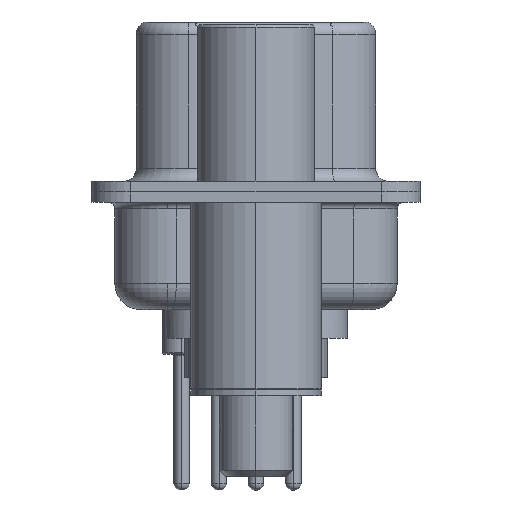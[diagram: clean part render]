
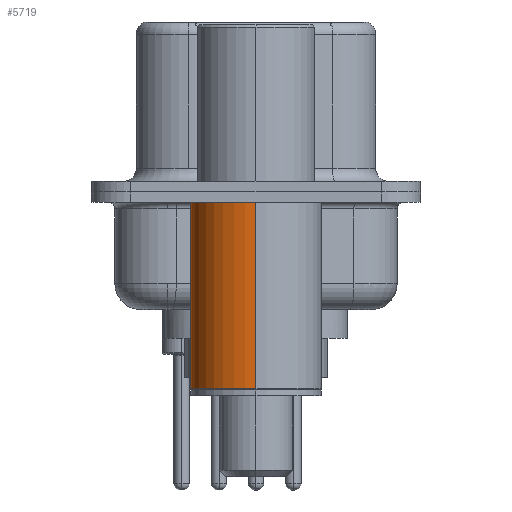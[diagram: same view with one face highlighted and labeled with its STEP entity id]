
A CAD part, left-side view. The second image highlights one B-rep face of the part: STEP entity #5719.
In plain terms, the highlighted cylindrical face has radius 2.5 mm (diameter 5 mm), a partial arc.
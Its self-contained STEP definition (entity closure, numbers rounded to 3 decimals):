
#463 = ORIENTED_EDGE ( 'NONE', *, *, #3000, .F. ) ;
#952 = DIRECTION ( 'NONE',  ( 0., 0., 1. ) ) ;
#1108 = CARTESIAN_POINT ( 'NONE',  ( 2.5, 0., 0.581 ) ) ;
#1246 = FACE_OUTER_BOUND ( 'NONE', #25234, .T. ) ;
#1771 = CIRCLE ( 'NONE', #19673, 2.5 ) ;
#1999 = VECTOR ( 'NONE', #24721, 1000. ) ;
#2652 = LINE ( 'NONE', #24866, #1999 ) ;
#2879 = DIRECTION ( 'NONE',  ( 1., 0., 0. ) ) ;
#3000 = EDGE_CURVE ( 'NONE', #19022, #24059, #10013, .T. ) ;
#3647 = DIRECTION ( 'NONE',  ( 1., 0., 0. ) ) ;
#4002 = EDGE_CURVE ( 'NONE', #20399, #24059, #2652, .T. ) ;
#4532 = EDGE_CURVE ( 'NONE', #15777, #19022, #20188, .T. ) ;
#5174 = CARTESIAN_POINT ( 'NONE',  ( 0., 0., -0.4 ) ) ;
#5719 = ADVANCED_FACE ( 'NONE', ( #1246 ), #17496, .T. ) ;
#7270 = CARTESIAN_POINT ( 'NONE',  ( 0., 0., -7.525 ) ) ;
#7713 = ORIENTED_EDGE ( 'NONE', *, *, #18188, .T. ) ;
#9398 = DIRECTION ( 'NONE',  ( 1., 0., 0. ) ) ;
#9495 = DIRECTION ( 'NONE',  ( 0., 0., 1. ) ) ;
#9958 = CARTESIAN_POINT ( 'NONE',  ( -2.5, 0., -7.525 ) ) ;
#10013 = CIRCLE ( 'NONE', #23961, 2.5 ) ;
#11691 = ORIENTED_EDGE ( 'NONE', *, *, #4532, .F. ) ;
#12220 = DIRECTION ( 'NONE',  ( 0., 0., 1. ) ) ;
#12671 = CARTESIAN_POINT ( 'NONE',  ( 2.5, 0., -0.4 ) ) ;
#15777 = VERTEX_POINT ( 'NONE', #18247 ) ;
#16660 = ORIENTED_EDGE ( 'NONE', *, *, #4002, .T. ) ;
#17496 = CYLINDRICAL_SURFACE ( 'NONE', #27222, 2.5 ) ;
#18188 = EDGE_CURVE ( 'NONE', #15777, #20399, #1771, .T. ) ;
#18247 = CARTESIAN_POINT ( 'NONE',  ( 2.5, 0., -7.525 ) ) ;
#18880 = VECTOR ( 'NONE', #952, 1000. ) ;
#19022 = VERTEX_POINT ( 'NONE', #12671 ) ;
#19673 = AXIS2_PLACEMENT_3D ( 'NONE', #7270, #22057, #9398 ) ;
#20188 = LINE ( 'NONE', #1108, #18880 ) ;
#20399 = VERTEX_POINT ( 'NONE', #9958 ) ;
#22057 = DIRECTION ( 'NONE',  ( 0., 0., 1. ) ) ;
#23961 = AXIS2_PLACEMENT_3D ( 'NONE', #5174, #9495, #2879 ) ;
#24059 = VERTEX_POINT ( 'NONE', #24140 ) ;
#24140 = CARTESIAN_POINT ( 'NONE',  ( -2.5, 0., -0.4 ) ) ;
#24721 = DIRECTION ( 'NONE',  ( 0., 0., 1. ) ) ;
#24866 = CARTESIAN_POINT ( 'NONE',  ( -2.5, 0., 0.581 ) ) ;
#25234 = EDGE_LOOP ( 'NONE', ( #7713, #16660, #463, #11691 ) ) ;
#26934 = CARTESIAN_POINT ( 'NONE',  ( 0., 0., 0.581 ) ) ;
#27222 = AXIS2_PLACEMENT_3D ( 'NONE', #26934, #12220, #3647 ) ;
